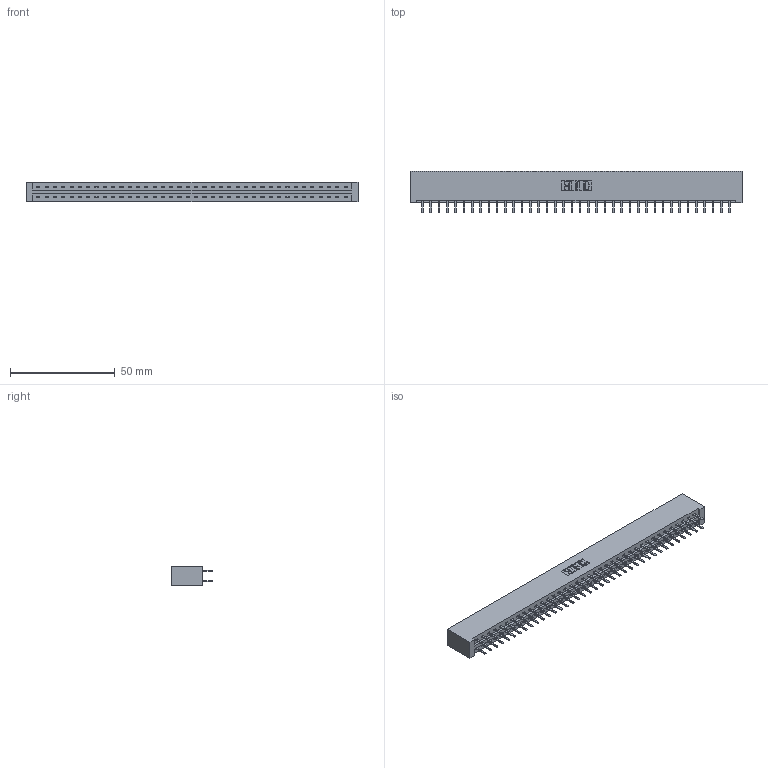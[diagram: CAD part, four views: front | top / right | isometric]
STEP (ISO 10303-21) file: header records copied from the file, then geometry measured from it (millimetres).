
FILE_DESCRIPTION (( 'STEP AP203' ), '1' );
FILE_NAME ('337-076-520-201.STEP', '2019-10-10T04:37:46', ( '' ), ( '' ), 'SwSTEP 2.0', 'SolidWorks 2016', '' );
FILE_SCHEMA (( 'CONFIG_CONTROL_DESIGN' ));
Length unit declared in the file: inch
Products named in the file (3): 337-076-520-201; 337 Part_No Mounting Lugs; 345-292-001_345-293-120
Assembly tree (77 placements, depth 2):
  337-076-520-201
    337 Part_No Mounting Lugs
    345-292-001_345-293-120  x76
Bounding box: 158.45 x 20.02 x 9.4 mm (x, y, z)
Volume: 17372.3 mm3; surface area: 19561.4 mm2
Topology: 77 solids, 77 shells, 4514 faces, 13131 edges, 8550 vertices
Faces by surface type: plane 3106, cylinder 1408
Entity records: 29817 total; most frequent: CARTESIAN_POINT 5038, ORIENTED_EDGE 4962, DIRECTION 4273, EDGE_CURVE 2481, LINE 2357, VECTOR 2357, VERTEX_POINT 1650, AXIS2_PLACEMENT_3D 958
